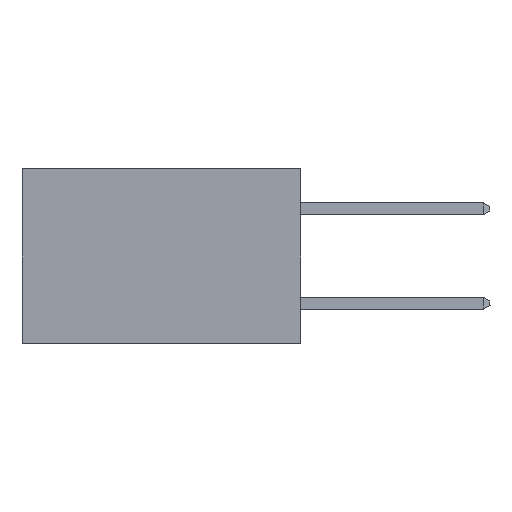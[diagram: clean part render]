
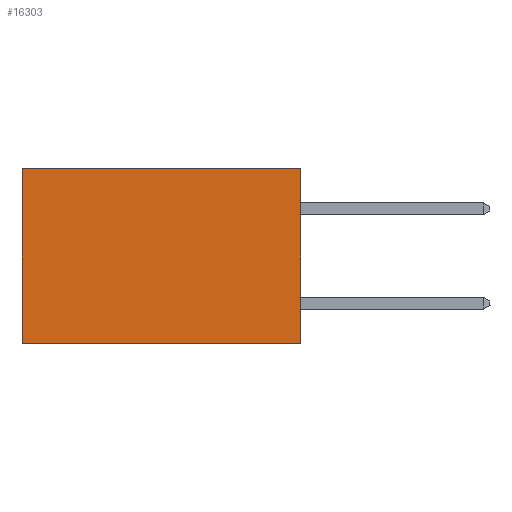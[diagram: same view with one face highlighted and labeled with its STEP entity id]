
A CAD part, left-side view. The second image highlights one B-rep face of the part: STEP entity #16303.
In plain terms, the highlighted planar face has unit normal (-1, 0, 0).
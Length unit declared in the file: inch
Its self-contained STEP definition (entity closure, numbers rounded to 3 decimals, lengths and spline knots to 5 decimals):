
#1574 = EDGE_CURVE ( 'NONE', #9975, #18250, #8247, .T. ) ;
#2619 = DIRECTION ( 'NONE',  ( 0., 0., -1. ) ) ;
#3225 = LINE ( 'NONE', #10389, #8471 ) ;
#3301 = VERTEX_POINT ( 'NONE', #23638 ) ;
#5910 = ORIENTED_EDGE ( 'NONE', *, *, #13266, .T. ) ;
#6598 = LINE ( 'NONE', #15573, #7417 ) ;
#7331 = EDGE_LOOP ( 'NONE', ( #9039, #24536, #24070, #5910 ) ) ;
#7417 = VECTOR ( 'NONE', #31014, 39.37008 ) ;
#8069 = DIRECTION ( 'NONE',  ( 0., 1., 0. ) ) ;
#8247 = LINE ( 'NONE', #16169, #15056 ) ;
#8471 = VECTOR ( 'NONE', #2619, 39.37008 ) ;
#9033 = CARTESIAN_POINT ( 'NONE',  ( 0.277, 0.59, 0. ) ) ;
#9039 = ORIENTED_EDGE ( 'NONE', *, *, #1574, .T. ) ;
#9975 = VERTEX_POINT ( 'NONE', #9033 ) ;
#10389 = CARTESIAN_POINT ( 'NONE',  ( 0.277, 0., -0.37 ) ) ;
#13266 = EDGE_CURVE ( 'NONE', #3301, #9975, #19904, .T. ) ;
#13311 = DIRECTION ( 'NONE',  ( 1., 0., 0. ) ) ;
#15056 = VECTOR ( 'NONE', #25180, 39.37008 ) ;
#15573 = CARTESIAN_POINT ( 'NONE',  ( 0.277, 0., -0.37 ) ) ;
#16169 = CARTESIAN_POINT ( 'NONE',  ( 0.277, 0.59, -0.37 ) ) ;
#16303 = ADVANCED_FACE ( 'NONE', ( #26466 ), #23632, .F. ) ;
#17735 = CARTESIAN_POINT ( 'NONE',  ( 0.277, 0.59, -0.37 ) ) ;
#18250 = VERTEX_POINT ( 'NONE', #17735 ) ;
#19094 = CARTESIAN_POINT ( 'NONE',  ( 0.277, 0., -0.37 ) ) ;
#19904 = LINE ( 'NONE', #26107, #26746 ) ;
#20373 = EDGE_CURVE ( 'NONE', #3301, #25671, #3225, .T. ) ;
#23632 = PLANE ( 'NONE',  #31348 ) ;
#23638 = CARTESIAN_POINT ( 'NONE',  ( 0.277, 0., 0. ) ) ;
#24070 = ORIENTED_EDGE ( 'NONE', *, *, #20373, .F. ) ;
#24536 = ORIENTED_EDGE ( 'NONE', *, *, #27528, .F. ) ;
#25180 = DIRECTION ( 'NONE',  ( 0., 0., -1. ) ) ;
#25671 = VERTEX_POINT ( 'NONE', #19094 ) ;
#26107 = CARTESIAN_POINT ( 'NONE',  ( 0.277, 0., 0. ) ) ;
#26466 = FACE_OUTER_BOUND ( 'NONE', #7331, .T. ) ;
#26746 = VECTOR ( 'NONE', #8069, 39.37008 ) ;
#27528 = EDGE_CURVE ( 'NONE', #25671, #18250, #6598, .T. ) ;
#28781 = CARTESIAN_POINT ( 'NONE',  ( 0.277, 0., -0.37 ) ) ;
#31014 = DIRECTION ( 'NONE',  ( 0., 1., 0. ) ) ;
#31326 = DIRECTION ( 'NONE',  ( 0., 0., -1. ) ) ;
#31348 = AXIS2_PLACEMENT_3D ( 'NONE', #28781, #13311, #31326 ) ;
